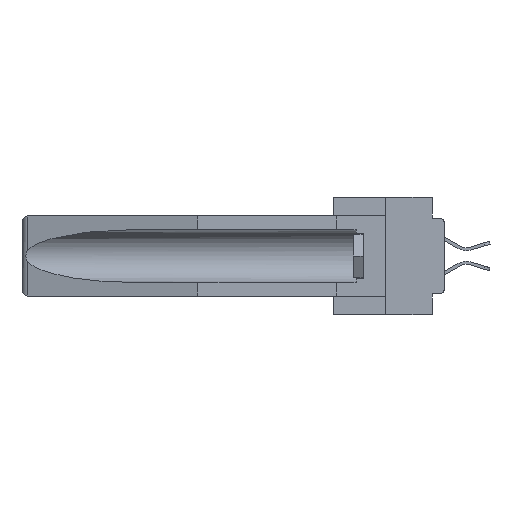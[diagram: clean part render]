
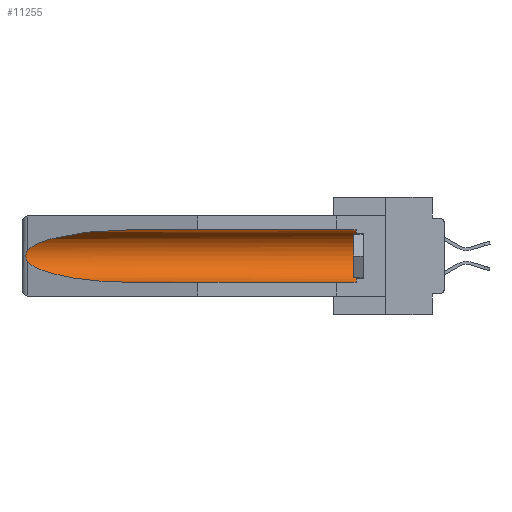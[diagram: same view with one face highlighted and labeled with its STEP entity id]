
A CAD part, left-side view. The second image highlights one B-rep face of the part: STEP entity #11255.
In plain terms, the highlighted cylindrical face has radius 2.857 mm (diameter 5.715 mm), a partial arc.
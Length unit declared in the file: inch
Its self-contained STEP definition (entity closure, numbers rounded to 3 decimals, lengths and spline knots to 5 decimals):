
#692 = CARTESIAN_POINT ( 'NONE',  ( 0.26537, 1.52718, -0.14972 ) ) ;
#821 = CARTESIAN_POINT ( 'NONE',  ( 0.155, 1.07973, -0.284 ) ) ;
#1513 = AXIS2_PLACEMENT_3D ( 'NONE', #22791, #3021, #12909 ) ;
#1736 = EDGE_LOOP ( 'NONE', ( #8626, #21688, #5718, #22401, #26087, #18416 ) ) ;
#1795 = CYLINDRICAL_SURFACE ( 'NONE', #2838, 0.1125 ) ;
#1869 = VERTEX_POINT ( 'NONE', #28240 ) ;
#2838 = AXIS2_PLACEMENT_3D ( 'NONE', #7733, #24699, #11863 ) ;
#3021 = DIRECTION ( 'NONE',  ( 0., -1., 0. ) ) ;
#3290 = CARTESIAN_POINT ( 'NONE',  ( 0.26537, 1.52718, -0.14972 ) ) ;
#4138 = CARTESIAN_POINT ( 'NONE',  ( 0.26597, 1.5296, -0.19026 ) ) ;
#4418 = VERTEX_POINT ( 'NONE', #11303 ) ;
#4637 =( BOUNDED_CURVE ( )  B_SPLINE_CURVE ( 3, ( #17880, #13027, #12602, #692 ),
 .UNSPECIFIED., .F., .F. ) 
 B_SPLINE_CURVE_WITH_KNOTS ( ( 4, 4 ),
 ( 4.71239, 6.08839 ),
 .UNSPECIFIED. ) 
 CURVE ( )  GEOMETRIC_REPRESENTATION_ITEM ( )  RATIONAL_B_SPLINE_CURVE ( ( 1., 0.848, 0.848, 1. ) ) 
 REPRESENTATION_ITEM ( '' )  );
#5203 = LINE ( 'NONE', #15482, #26096 ) ;
#5718 = ORIENTED_EDGE ( 'NONE', *, *, #28430, .T. ) ;
#6487 = CARTESIAN_POINT ( 'NONE',  ( 0.2675, 1.53308, -0.17534 ) ) ;
#6602 = VERTEX_POINT ( 'NONE', #22170 ) ;
#6650 = VERTEX_POINT ( 'NONE', #12620 ) ;
#6692 = CARTESIAN_POINT ( 'NONE',  ( 0.2673, 1.53269, -0.17917 ) ) ;
#7298 = CIRCLE ( 'NONE', #1513, 0.1125 ) ;
#7733 = CARTESIAN_POINT ( 'NONE',  ( 0.155, -0.30754, -0.1715 ) ) ;
#7766 = EDGE_CURVE ( 'NONE', #6650, #6602, #30549, .T. ) ;
#8248 = EDGE_CURVE ( 'NONE', #4418, #1869, #24700, .T. ) ;
#8626 = ORIENTED_EDGE ( 'NONE', *, *, #11322, .T. ) ;
#8654 = CARTESIAN_POINT ( 'NONE',  ( 0.155, -0.30754, -0.059 ) ) ;
#8835 = CARTESIAN_POINT ( 'NONE',  ( 0.26654, 1.53092, -0.15636 ) ) ;
#11255 = ADVANCED_FACE ( 'NONE', ( #14357 ), #1795, .F. ) ;
#11303 = CARTESIAN_POINT ( 'NONE',  ( 0.155, 0.126, -0.059 ) ) ;
#11322 = EDGE_CURVE ( 'NONE', #1869, #6650, #4637, .T. ) ;
#11370 = CARTESIAN_POINT ( 'NONE',  ( 0.26655, 1.53094, -0.18657 ) ) ;
#11863 = DIRECTION ( 'NONE',  ( 0., 0., 1. ) ) ;
#12016 = EDGE_CURVE ( 'NONE', #30145, #30473, #5203, .T. ) ;
#12602 = CARTESIAN_POINT ( 'NONE',  ( 0.25451, 1.48313, -0.09465 ) ) ;
#12620 = CARTESIAN_POINT ( 'NONE',  ( 0.26537, 1.52718, -0.14972 ) ) ;
#12909 = DIRECTION ( 'NONE',  ( 0., 0., 1. ) ) ;
#13027 = CARTESIAN_POINT ( 'NONE',  ( 0.21114, 1.30732, -0.059 ) ) ;
#13063 = CARTESIAN_POINT ( 'NONE',  ( 0.155, 1.07973, -0.284 ) ) ;
#13599 = DIRECTION ( 'NONE',  ( 0., 1., 0. ) ) ;
#14357 = FACE_OUTER_BOUND ( 'NONE', #1736, .T. ) ;
#15000 = EDGE_CURVE ( 'NONE', #30145, #4418, #7298, .T. ) ;
#15482 = CARTESIAN_POINT ( 'NONE',  ( 0.155, -0.30754, -0.284 ) ) ;
#15579 = CARTESIAN_POINT ( 'NONE',  ( 0.25451, 1.48313, -0.24835 ) ) ;
#17880 = CARTESIAN_POINT ( 'NONE',  ( 0.155, 1.07973, -0.059 ) ) ;
#18416 = ORIENTED_EDGE ( 'NONE', *, *, #8248, .T. ) ;
#18676 = CARTESIAN_POINT ( 'NONE',  ( 0.2675, 1.53308, -0.16763 ) ) ;
#20915 = CARTESIAN_POINT ( 'NONE',  ( 0.26597, 1.52961, -0.15275 ) ) ;
#21688 = ORIENTED_EDGE ( 'NONE', *, *, #7766, .T. ) ;
#22170 = CARTESIAN_POINT ( 'NONE',  ( 0.26537, 1.52718, -0.19328 ) ) ;
#22401 = ORIENTED_EDGE ( 'NONE', *, *, #12016, .F. ) ;
#22791 = CARTESIAN_POINT ( 'NONE',  ( 0.155, 0.126, -0.1715 ) ) ;
#23598 = CARTESIAN_POINT ( 'NONE',  ( 0.26537, 1.52718, -0.19328 ) ) ;
#23968 = VECTOR ( 'NONE', #28258, 39.37008 ) ;
#24699 = DIRECTION ( 'NONE',  ( 0., 1., 0. ) ) ;
#24700 = LINE ( 'NONE', #8654, #23968 ) ;
#25136 = CARTESIAN_POINT ( 'NONE',  ( 0.21114, 1.30732, -0.284 ) ) ;
#25792 = CARTESIAN_POINT ( 'NONE',  ( 0.2673, 1.5327, -0.16383 ) ) ;
#26087 = ORIENTED_EDGE ( 'NONE', *, *, #15000, .T. ) ;
#26096 = VECTOR ( 'NONE', #13599, 39.37008 ) ;
#26755 = CARTESIAN_POINT ( 'NONE',  ( 0.155, 0.126, -0.284 ) ) ;
#26823 =( BOUNDED_CURVE ( )  B_SPLINE_CURVE ( 3, ( #30142, #15579, #25136, #821 ),
 .UNSPECIFIED., .F., .T. ) 
 B_SPLINE_CURVE_WITH_KNOTS ( ( 4, 4 ),
 ( 0.1948, 1.5708 ),
 .UNSPECIFIED. ) 
 CURVE ( )  GEOMETRIC_REPRESENTATION_ITEM ( )  RATIONAL_B_SPLINE_CURVE ( ( 1., 0.848, 0.848, 1. ) ) 
 REPRESENTATION_ITEM ( '' )  );
#28240 = CARTESIAN_POINT ( 'NONE',  ( 0.155, 1.07973, -0.059 ) ) ;
#28258 = DIRECTION ( 'NONE',  ( 0., 1., 0. ) ) ;
#28430 = EDGE_CURVE ( 'NONE', #6602, #30473, #26823, .T. ) ;
#30142 = CARTESIAN_POINT ( 'NONE',  ( 0.26537, 1.52718, -0.19328 ) ) ;
#30145 = VERTEX_POINT ( 'NONE', #26755 ) ;
#30473 = VERTEX_POINT ( 'NONE', #13063 ) ;
#30549 = B_SPLINE_CURVE_WITH_KNOTS ( 'NONE', 3,
 ( #3290, #20915, #8835, #25792, #18676, #6487, #6692, #11370, #4138, #23598 ),
 .UNSPECIFIED., .F., .F.,
 ( 4, 2, 2, 2, 4 ),
 ( 0., 0.00029, 0.00058, 0.00087, 0.00117 ),
 .UNSPECIFIED. ) ;
